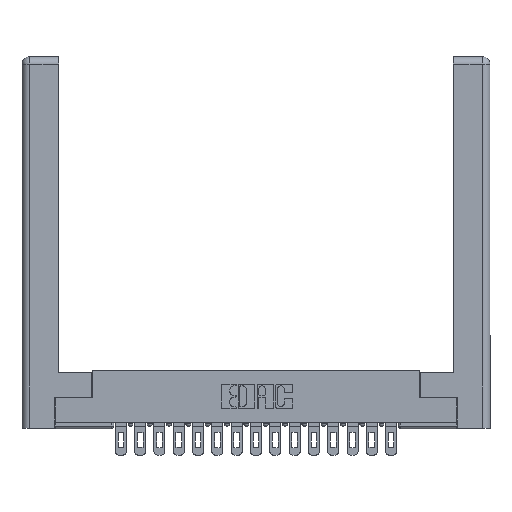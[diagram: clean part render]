
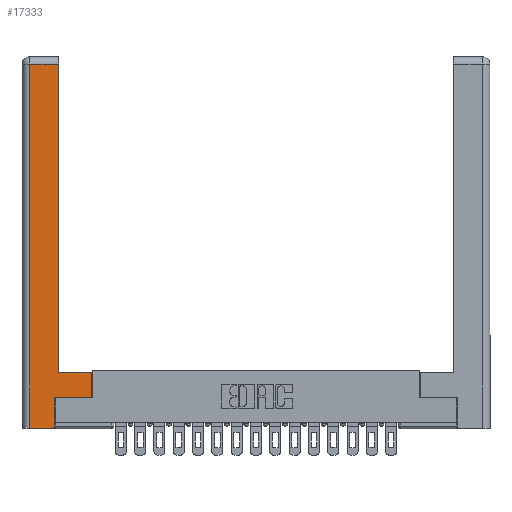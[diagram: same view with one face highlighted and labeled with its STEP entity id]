
A CAD part, top view. The second image highlights one B-rep face of the part: STEP entity #17333.
In plain terms, the highlighted planar face has unit normal (0, 0, 1).
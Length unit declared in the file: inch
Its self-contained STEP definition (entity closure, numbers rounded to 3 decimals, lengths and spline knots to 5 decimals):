
#116 = LINE ( 'NONE', #4873, #6716 ) ;
#463 = LINE ( 'NONE', #3343, #9719 ) ;
#1109 = DIRECTION ( 'NONE',  ( 0., 1., 0. ) ) ;
#1149 = DIRECTION ( 'NONE',  ( 1., 0., 0. ) ) ;
#1821 = VECTOR ( 'NONE', #2740, 39.37008 ) ;
#2337 = EDGE_CURVE ( 'NONE', #16998, #5941, #463, .T. ) ;
#2520 = VECTOR ( 'NONE', #1109, 39.37008 ) ;
#2740 = DIRECTION ( 'NONE',  ( -1., 0., 0. ) ) ;
#3343 = CARTESIAN_POINT ( 'NONE',  ( 0.565, 0.45, 0. ) ) ;
#3914 = ORIENTED_EDGE ( 'NONE', *, *, #4606, .T. ) ;
#3990 = CARTESIAN_POINT ( 'NONE',  ( 0.565, 0.245, 0. ) ) ;
#4225 = LINE ( 'NONE', #19318, #9056 ) ;
#4229 = VECTOR ( 'NONE', #14358, 39.37008 ) ;
#4466 = ORIENTED_EDGE ( 'NONE', *, *, #11441, .T. ) ;
#4482 = VERTEX_POINT ( 'NONE', #11762 ) ;
#4606 = EDGE_CURVE ( 'NONE', #19244, #6558, #15714, .T. ) ;
#4873 = CARTESIAN_POINT ( 'NONE',  ( 0.0615, 0., 0. ) ) ;
#4911 = EDGE_CURVE ( 'NONE', #14278, #4482, #116, .T. ) ;
#5779 = LINE ( 'NONE', #7373, #2520 ) ;
#5941 = VERTEX_POINT ( 'NONE', #7154 ) ;
#6388 = VECTOR ( 'NONE', #17613, 39.37008 ) ;
#6558 = VERTEX_POINT ( 'NONE', #12168 ) ;
#6716 = VECTOR ( 'NONE', #18293, 39.37008 ) ;
#6814 = VECTOR ( 'NONE', #9040, 39.37008 ) ;
#7154 = CARTESIAN_POINT ( 'NONE',  ( 0.565, 0.45, 0. ) ) ;
#7165 = LINE ( 'NONE', #10530, #6814 ) ;
#7373 = CARTESIAN_POINT ( 'NONE',  ( 0.295, 3., 0. ) ) ;
#7484 = ORIENTED_EDGE ( 'NONE', *, *, #18423, .T. ) ;
#7673 = ORIENTED_EDGE ( 'NONE', *, *, #2337, .T. ) ;
#8114 = EDGE_CURVE ( 'NONE', #4482, #19244, #11476, .T. ) ;
#8131 = PLANE ( 'NONE',  #9190 ) ;
#9040 = DIRECTION ( 'NONE',  ( -1., 0., 0. ) ) ;
#9056 = VECTOR ( 'NONE', #1149, 39.37008 ) ;
#9093 = EDGE_CURVE ( 'NONE', #5941, #14261, #7165, .T. ) ;
#9190 = AXIS2_PLACEMENT_3D ( 'NONE', #14395, #18969, #17578 ) ;
#9719 = VECTOR ( 'NONE', #17155, 39.37008 ) ;
#10530 = CARTESIAN_POINT ( 'NONE',  ( 0.295, 0.45, 0. ) ) ;
#11441 = EDGE_CURVE ( 'NONE', #6558, #16998, #4225, .T. ) ;
#11476 = LINE ( 'NONE', #11570, #4229 ) ;
#11570 = CARTESIAN_POINT ( 'NONE',  ( 0.265, 0., 0. ) ) ;
#11762 = CARTESIAN_POINT ( 'NONE',  ( 0.0615, 0., 0. ) ) ;
#12168 = CARTESIAN_POINT ( 'NONE',  ( 0.265, 0.245, 0. ) ) ;
#13037 = ORIENTED_EDGE ( 'NONE', *, *, #8114, .T. ) ;
#13200 = CARTESIAN_POINT ( 'NONE',  ( 0.295, 2.94, 0. ) ) ;
#13301 = ORIENTED_EDGE ( 'NONE', *, *, #9093, .T. ) ;
#13468 = LINE ( 'NONE', #14855, #1821 ) ;
#14261 = VERTEX_POINT ( 'NONE', #15221 ) ;
#14278 = VERTEX_POINT ( 'NONE', #18302 ) ;
#14358 = DIRECTION ( 'NONE',  ( 1., 0., 0. ) ) ;
#14395 = CARTESIAN_POINT ( 'NONE',  ( 0., 0., 0. ) ) ;
#14855 = CARTESIAN_POINT ( 'NONE',  ( 0.0615, 2.94, 0. ) ) ;
#14908 = CARTESIAN_POINT ( 'NONE',  ( 0.265, 0., 0. ) ) ;
#15221 = CARTESIAN_POINT ( 'NONE',  ( 0.295, 0.45, 0. ) ) ;
#15585 = FACE_OUTER_BOUND ( 'NONE', #16986, .T. ) ;
#15714 = LINE ( 'NONE', #17313, #6388 ) ;
#15936 = ORIENTED_EDGE ( 'NONE', *, *, #4911, .T. ) ;
#16986 = EDGE_LOOP ( 'NONE', ( #17611, #7484, #15936, #13037, #3914, #4466, #7673, #13301 ) ) ;
#16998 = VERTEX_POINT ( 'NONE', #3990 ) ;
#17058 = EDGE_CURVE ( 'NONE', #14261, #17463, #5779, .T. ) ;
#17155 = DIRECTION ( 'NONE',  ( 0., 1., 0. ) ) ;
#17313 = CARTESIAN_POINT ( 'NONE',  ( 0.265, 0.245, 0. ) ) ;
#17333 = ADVANCED_FACE ( 'NONE', ( #15585 ), #8131, .F. ) ;
#17463 = VERTEX_POINT ( 'NONE', #13200 ) ;
#17578 = DIRECTION ( 'NONE',  ( -1., 0., 0. ) ) ;
#17611 = ORIENTED_EDGE ( 'NONE', *, *, #17058, .T. ) ;
#17613 = DIRECTION ( 'NONE',  ( 0., 1., 0. ) ) ;
#18293 = DIRECTION ( 'NONE',  ( 0., -1., 0. ) ) ;
#18302 = CARTESIAN_POINT ( 'NONE',  ( 0.0615, 2.94, 0. ) ) ;
#18423 = EDGE_CURVE ( 'NONE', #17463, #14278, #13468, .T. ) ;
#18969 = DIRECTION ( 'NONE',  ( 0., 0., -1. ) ) ;
#19244 = VERTEX_POINT ( 'NONE', #14908 ) ;
#19318 = CARTESIAN_POINT ( 'NONE',  ( 0.565, 0.245, 0. ) ) ;
